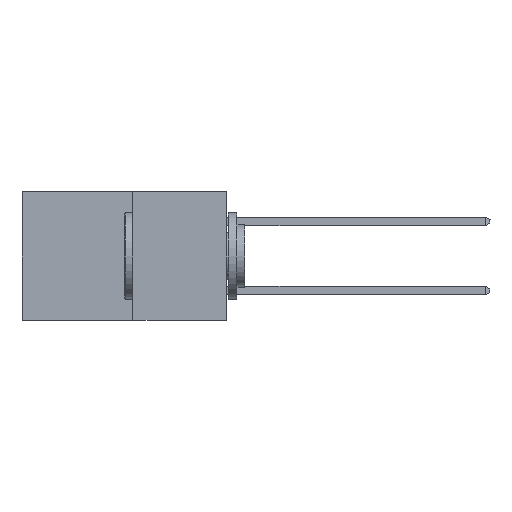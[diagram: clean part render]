
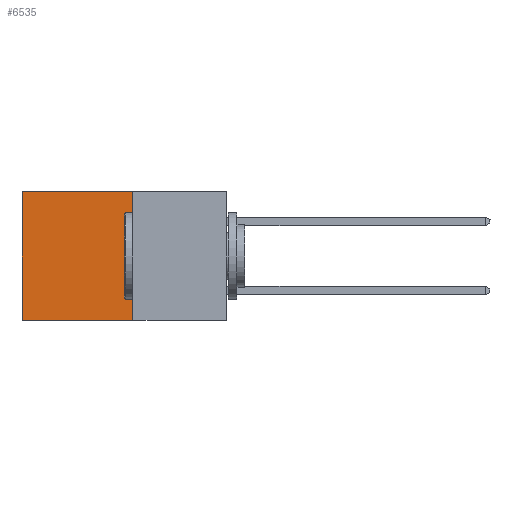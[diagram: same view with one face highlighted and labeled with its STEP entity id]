
A CAD part, left-side view. The second image highlights one B-rep face of the part: STEP entity #6535.
In plain terms, the highlighted planar face has unit normal (-1, 0, 0).
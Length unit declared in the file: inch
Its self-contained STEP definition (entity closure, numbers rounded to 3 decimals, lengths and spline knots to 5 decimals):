
#309 = CARTESIAN_POINT ( 'NONE',  ( 0.277, 0.27, -0.37 ) ) ;
#439 = CARTESIAN_POINT ( 'NONE',  ( 0.277, 0.27, 0. ) ) ;
#936 = DIRECTION ( 'NONE',  ( 0., 0., -1. ) ) ;
#1414 = DIRECTION ( 'NONE',  ( 0., 0., -1. ) ) ;
#1968 = LINE ( 'NONE', #10221, #18143 ) ;
#3354 = FACE_OUTER_BOUND ( 'NONE', #27941, .T. ) ;
#3371 = LINE ( 'NONE', #16084, #16795 ) ;
#5474 = CARTESIAN_POINT ( 'NONE',  ( 0.277, 0.59, 0. ) ) ;
#6129 = VERTEX_POINT ( 'NONE', #5474 ) ;
#6223 = ORIENTED_EDGE ( 'NONE', *, *, #11842, .T. ) ;
#6535 = ADVANCED_FACE ( 'NONE', ( #3354 ), #19763, .F. ) ;
#6996 = EDGE_CURVE ( 'NONE', #24331, #13465, #32300, .T. ) ;
#7769 = VECTOR ( 'NONE', #1414, 39.37008 ) ;
#10221 = CARTESIAN_POINT ( 'NONE',  ( 0.277, 0.27, 0. ) ) ;
#11587 = CARTESIAN_POINT ( 'NONE',  ( 0.277, 0.59, -0.37 ) ) ;
#11842 = EDGE_CURVE ( 'NONE', #6129, #13465, #3371, .T. ) ;
#12750 = DIRECTION ( 'NONE',  ( 0., 1., 0. ) ) ;
#13465 = VERTEX_POINT ( 'NONE', #11587 ) ;
#13645 = LINE ( 'NONE', #16572, #7769 ) ;
#13855 = ORIENTED_EDGE ( 'NONE', *, *, #30910, .T. ) ;
#15557 = CARTESIAN_POINT ( 'NONE',  ( 0.277, 0.27, -0.37 ) ) ;
#16084 = CARTESIAN_POINT ( 'NONE',  ( 0.277, 0.59, -0.37 ) ) ;
#16572 = CARTESIAN_POINT ( 'NONE',  ( 0.277, 0.27, -0.37 ) ) ;
#16795 = VECTOR ( 'NONE', #936, 39.37008 ) ;
#18143 = VECTOR ( 'NONE', #12750, 39.37008 ) ;
#19153 = AXIS2_PLACEMENT_3D ( 'NONE', #19917, #19540, #19321 ) ;
#19321 = DIRECTION ( 'NONE',  ( 0., 0., -1. ) ) ;
#19540 = DIRECTION ( 'NONE',  ( 1., 0., 0. ) ) ;
#19598 = EDGE_CURVE ( 'NONE', #20779, #24331, #13645, .T. ) ;
#19763 = PLANE ( 'NONE',  #19153 ) ;
#19917 = CARTESIAN_POINT ( 'NONE',  ( 0.277, 0.27, -0.37 ) ) ;
#20779 = VERTEX_POINT ( 'NONE', #439 ) ;
#24057 = ORIENTED_EDGE ( 'NONE', *, *, #19598, .F. ) ;
#24331 = VERTEX_POINT ( 'NONE', #15557 ) ;
#25073 = ORIENTED_EDGE ( 'NONE', *, *, #6996, .F. ) ;
#25743 = VECTOR ( 'NONE', #31755, 39.37008 ) ;
#27941 = EDGE_LOOP ( 'NONE', ( #6223, #25073, #24057, #13855 ) ) ;
#30910 = EDGE_CURVE ( 'NONE', #20779, #6129, #1968, .T. ) ;
#31755 = DIRECTION ( 'NONE',  ( 0., 1., 0. ) ) ;
#32300 = LINE ( 'NONE', #309, #25743 ) ;
